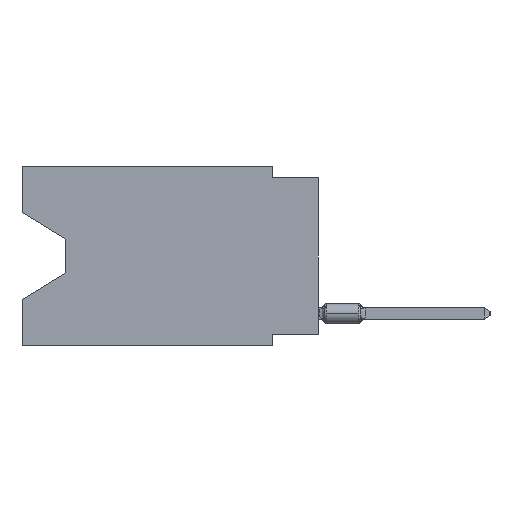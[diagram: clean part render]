
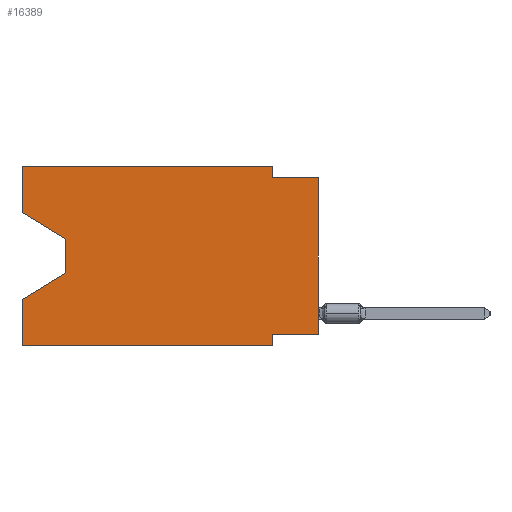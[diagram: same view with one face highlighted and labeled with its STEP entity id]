
A CAD part, left-side view. The second image highlights one B-rep face of the part: STEP entity #16389.
In plain terms, the highlighted planar face has unit normal (-1, 0, 0).
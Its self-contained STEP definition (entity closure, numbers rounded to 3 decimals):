
#36 = CARTESIAN_POINT ( 'NONE',  ( 0., 16.383, -2.546 ) ) ;
#1555 = CARTESIAN_POINT ( 'NONE',  ( 0., 13.97, -4.013 ) ) ;
#1631 = LINE ( 'NONE', #10103, #27386 ) ;
#1887 = VECTOR ( 'NONE', #11881, 1000. ) ;
#2324 = VERTEX_POINT ( 'NONE', #10359 ) ;
#2367 = DIRECTION ( 'NONE',  ( 0., 0., 1. ) ) ;
#2869 = VERTEX_POINT ( 'NONE', #26873 ) ;
#3026 = ORIENTED_EDGE ( 'NONE', *, *, #11235, .F. ) ;
#3055 = CARTESIAN_POINT ( 'NONE',  ( 0., 13.97, -5.893 ) ) ;
#3411 = CARTESIAN_POINT ( 'NONE',  ( 0., 0., -0.635 ) ) ;
#3801 = VECTOR ( 'NONE', #20099, 1000. ) ;
#4448 = CARTESIAN_POINT ( 'NONE',  ( 0., 0., -0.635 ) ) ;
#4569 = CARTESIAN_POINT ( 'NONE',  ( 0., 16.383, -7.36 ) ) ;
#4878 = VERTEX_POINT ( 'NONE', #7458 ) ;
#5798 = CARTESIAN_POINT ( 'NONE',  ( 0., 16.383, -9.906 ) ) ;
#5903 = CARTESIAN_POINT ( 'NONE',  ( 0., 16.383, 0. ) ) ;
#6235 = ORIENTED_EDGE ( 'NONE', *, *, #15178, .T. ) ;
#6398 = DIRECTION ( 'NONE',  ( 0., 0., 1. ) ) ;
#6497 = VERTEX_POINT ( 'NONE', #16105 ) ;
#6666 = VERTEX_POINT ( 'NONE', #5798 ) ;
#6736 = EDGE_CURVE ( 'NONE', #19005, #22998, #20867, .T. ) ;
#7458 = CARTESIAN_POINT ( 'NONE',  ( 0., 2.54, -9.271 ) ) ;
#7843 = DIRECTION ( 'NONE',  ( 0., 1., 0. ) ) ;
#7981 = VECTOR ( 'NONE', #10170, 1000. ) ;
#7991 = CARTESIAN_POINT ( 'NONE',  ( 0., 16.383, -2.546 ) ) ;
#7995 = CARTESIAN_POINT ( 'NONE',  ( 0., 2.54, 0. ) ) ;
#8120 = DIRECTION ( 'NONE',  ( 0., -0.855, -0.519 ) ) ;
#8220 = DIRECTION ( 'NONE',  ( 0., -1., 0. ) ) ;
#8361 = ORIENTED_EDGE ( 'NONE', *, *, #8557, .F. ) ;
#8557 = EDGE_CURVE ( 'NONE', #2324, #4878, #1631, .T. ) ;
#9309 = AXIS2_PLACEMENT_3D ( 'NONE', #5903, #14495, #23090 ) ;
#9413 = DIRECTION ( 'NONE',  ( 0., 0.855, -0.519 ) ) ;
#10103 = CARTESIAN_POINT ( 'NONE',  ( 0., 0., -9.271 ) ) ;
#10114 = DIRECTION ( 'NONE',  ( 0., 0., -1. ) ) ;
#10170 = DIRECTION ( 'NONE',  ( 0., 0., -1. ) ) ;
#10359 = CARTESIAN_POINT ( 'NONE',  ( 0., 0., -9.271 ) ) ;
#10846 = CARTESIAN_POINT ( 'NONE',  ( 0., 0., 0. ) ) ;
#11085 = CARTESIAN_POINT ( 'NONE',  ( 0., 16.383, 0. ) ) ;
#11229 = LINE ( 'NONE', #11085, #3801 ) ;
#11235 = EDGE_CURVE ( 'NONE', #25878, #2869, #11229, .T. ) ;
#11881 = DIRECTION ( 'NONE',  ( 0., -1., 0. ) ) ;
#12106 = EDGE_CURVE ( 'NONE', #22998, #15298, #19839, .T. ) ;
#12582 = CARTESIAN_POINT ( 'NONE',  ( 0., 13.97, -4.013 ) ) ;
#12612 = ORIENTED_EDGE ( 'NONE', *, *, #22860, .F. ) ;
#13258 = ORIENTED_EDGE ( 'NONE', *, *, #12106, .T. ) ;
#13605 = DIRECTION ( 'NONE',  ( 0., 0., -1. ) ) ;
#13743 = EDGE_CURVE ( 'NONE', #6666, #25742, #18937, .T. ) ;
#13813 = VECTOR ( 'NONE', #13605, 1000. ) ;
#13961 = ORIENTED_EDGE ( 'NONE', *, *, #14772, .F. ) ;
#14454 = EDGE_CURVE ( 'NONE', #6497, #25340, #18700, .T. ) ;
#14495 = DIRECTION ( 'NONE',  ( 1., 0., 0. ) ) ;
#14642 = VECTOR ( 'NONE', #8220, 1000. ) ;
#14699 = VERTEX_POINT ( 'NONE', #4448 ) ;
#14772 = EDGE_CURVE ( 'NONE', #2869, #6497, #20223, .T. ) ;
#15122 = ORIENTED_EDGE ( 'NONE', *, *, #13743, .T. ) ;
#15178 = EDGE_CURVE ( 'NONE', #25878, #19005, #21097, .T. ) ;
#15298 = VERTEX_POINT ( 'NONE', #4569 ) ;
#15351 = LINE ( 'NONE', #10846, #24509 ) ;
#15613 = ORIENTED_EDGE ( 'NONE', *, *, #20735, .T. ) ;
#15720 = CARTESIAN_POINT ( 'NONE',  ( 0., 16.383, 0. ) ) ;
#16105 = CARTESIAN_POINT ( 'NONE',  ( 0., 2.54, 0. ) ) ;
#16254 = ORIENTED_EDGE ( 'NONE', *, *, #14454, .F. ) ;
#16389 = ADVANCED_FACE ( 'NONE', ( #20842 ), #18733, .F. ) ;
#16638 = CARTESIAN_POINT ( 'NONE',  ( 0., 2.54, -0.635 ) ) ;
#17389 = CARTESIAN_POINT ( 'NONE',  ( 0., 16.383, 0. ) ) ;
#17777 = ORIENTED_EDGE ( 'NONE', *, *, #21458, .F. ) ;
#18314 = VECTOR ( 'NONE', #10114, 1000. ) ;
#18662 = EDGE_LOOP ( 'NONE', ( #6235, #21562, #13258, #21024, #15122, #17777, #8361, #15613, #12612, #16254, #13961, #3026 ) ) ;
#18700 = LINE ( 'NONE', #7995, #18314 ) ;
#18733 = PLANE ( 'NONE',  #9309 ) ;
#18937 = LINE ( 'NONE', #27521, #14642 ) ;
#19005 = VERTEX_POINT ( 'NONE', #12582 ) ;
#19839 = LINE ( 'NONE', #3055, #25345 ) ;
#19948 = CARTESIAN_POINT ( 'NONE',  ( 0., 2.54, -9.906 ) ) ;
#20099 = DIRECTION ( 'NONE',  ( 0., 0., 1. ) ) ;
#20223 = LINE ( 'NONE', #15720, #26406 ) ;
#20513 = LINE ( 'NONE', #19948, #13813 ) ;
#20735 = EDGE_CURVE ( 'NONE', #2324, #14699, #15351, .T. ) ;
#20842 = FACE_OUTER_BOUND ( 'NONE', #18662, .T. ) ;
#20867 = LINE ( 'NONE', #1555, #7981 ) ;
#21024 = ORIENTED_EDGE ( 'NONE', *, *, #26000, .F. ) ;
#21097 = LINE ( 'NONE', #7991, #24933 ) ;
#21458 = EDGE_CURVE ( 'NONE', #4878, #25742, #20513, .T. ) ;
#21562 = ORIENTED_EDGE ( 'NONE', *, *, #6736, .T. ) ;
#21815 = CARTESIAN_POINT ( 'NONE',  ( 0., 2.54, -9.906 ) ) ;
#22172 = VECTOR ( 'NONE', #6398, 1000. ) ;
#22183 = DIRECTION ( 'NONE',  ( 0., -1., 0. ) ) ;
#22860 = EDGE_CURVE ( 'NONE', #25340, #14699, #27888, .T. ) ;
#22998 = VERTEX_POINT ( 'NONE', #24156 ) ;
#23090 = DIRECTION ( 'NONE',  ( 0., 0., -1. ) ) ;
#24156 = CARTESIAN_POINT ( 'NONE',  ( 0., 13.97, -5.893 ) ) ;
#24509 = VECTOR ( 'NONE', #2367, 1000. ) ;
#24933 = VECTOR ( 'NONE', #8120, 1000. ) ;
#25340 = VERTEX_POINT ( 'NONE', #16638 ) ;
#25345 = VECTOR ( 'NONE', #9413, 1000. ) ;
#25702 = LINE ( 'NONE', #17389, #22172 ) ;
#25742 = VERTEX_POINT ( 'NONE', #21815 ) ;
#25878 = VERTEX_POINT ( 'NONE', #36 ) ;
#26000 = EDGE_CURVE ( 'NONE', #6666, #15298, #25702, .T. ) ;
#26406 = VECTOR ( 'NONE', #22183, 1000. ) ;
#26873 = CARTESIAN_POINT ( 'NONE',  ( 0., 16.383, 0. ) ) ;
#27386 = VECTOR ( 'NONE', #7843, 1000. ) ;
#27521 = CARTESIAN_POINT ( 'NONE',  ( 0., 16.383, -9.906 ) ) ;
#27888 = LINE ( 'NONE', #3411, #1887 ) ;
